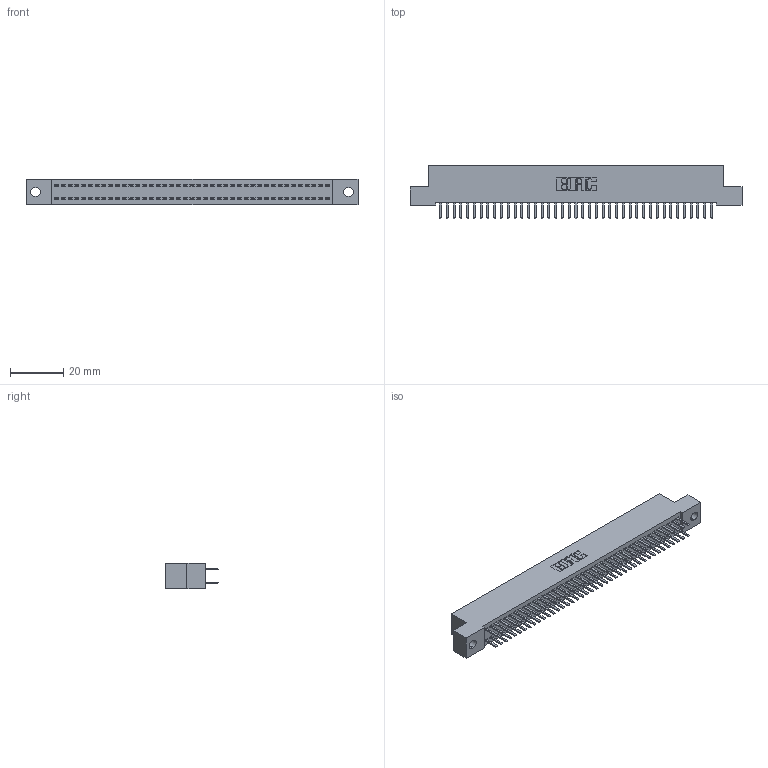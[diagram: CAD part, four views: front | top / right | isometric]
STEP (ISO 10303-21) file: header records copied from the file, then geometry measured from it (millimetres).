
FILE_DESCRIPTION (( 'STEP AP203' ), '1' );
FILE_NAME ('342-082-520-202.STEP', '2019-10-04T11:58:39', ( '' ), ( '' ), 'SwSTEP 2.0', 'SolidWorks 2016', '' );
FILE_SCHEMA (( 'CONFIG_CONTROL_DESIGN' ));
Length unit declared in the file: inch
Products named in the file (3): 342 Part_.128 Slot; 345-292-001_345-293-120; 342-082-520-202
Assembly tree (83 placements, depth 2):
  342-082-520-202
    342 Part_.128 Slot
    345-292-001_345-293-120  x82
Bounding box: 124.46 x 20.02 x 9.4 mm (x, y, z)
Volume: 11089.8 mm3; surface area: 17701.2 mm2
Topology: 83 solids, 83 shells, 4706 faces, 13677 edges, 8898 vertices
Faces by surface type: plane 3186, cylinder 1520
Entity records: 26623 total; most frequent: CARTESIAN_POINT 4426, ORIENTED_EDGE 4350, DIRECTION 3771, EDGE_CURVE 2175, LINE 2043, VECTOR 2043, VERTEX_POINT 1446, AXIS2_PLACEMENT_3D 864
